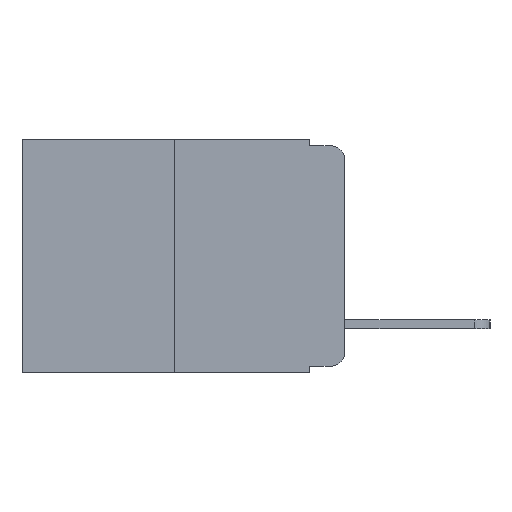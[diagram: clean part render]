
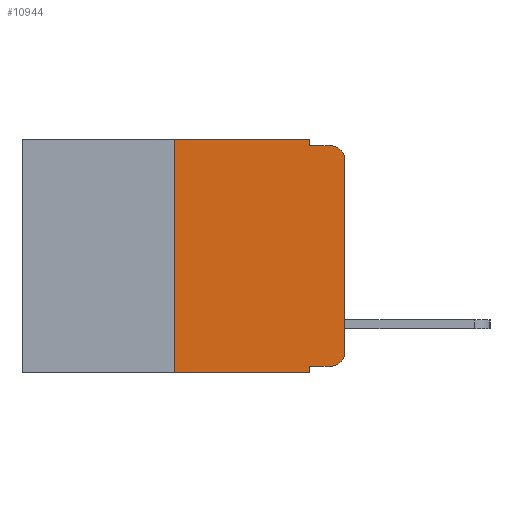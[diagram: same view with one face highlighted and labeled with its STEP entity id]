
A CAD part, left-side view. The second image highlights one B-rep face of the part: STEP entity #10944.
In plain terms, the highlighted planar face has unit normal (-1, 0, 0).
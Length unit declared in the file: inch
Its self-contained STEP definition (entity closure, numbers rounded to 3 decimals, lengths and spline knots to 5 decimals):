
#168 = ORIENTED_EDGE ( 'NONE', *, *, #9440, .F. ) ;
#286 = VERTEX_POINT ( 'NONE', #8980 ) ;
#292 = ORIENTED_EDGE ( 'NONE', *, *, #3671, .F. ) ;
#321 = LINE ( 'NONE', #7393, #3184 ) ;
#363 = VERTEX_POINT ( 'NONE', #466 ) ;
#466 = CARTESIAN_POINT ( 'NONE',  ( 0., 0.051, 0. ) ) ;
#645 = VERTEX_POINT ( 'NONE', #10876 ) ;
#827 = LINE ( 'NONE', #9065, #7703 ) ;
#958 = ORIENTED_EDGE ( 'NONE', *, *, #8987, .T. ) ;
#1052 = ORIENTED_EDGE ( 'NONE', *, *, #4785, .F. ) ;
#1501 = ORIENTED_EDGE ( 'NONE', *, *, #6517, .T. ) ;
#1769 = AXIS2_PLACEMENT_3D ( 'NONE', #6412, #6434, #8892 ) ;
#1824 = ORIENTED_EDGE ( 'NONE', *, *, #7734, .F. ) ;
#2064 = DIRECTION ( 'NONE',  ( 0., 0., -1. ) ) ;
#2206 = LINE ( 'NONE', #8111, #6698 ) ;
#2406 = EDGE_CURVE ( 'NONE', #8271, #8794, #7640, .T. ) ;
#2451 = PLANE ( 'NONE',  #5122 ) ;
#2508 = AXIS2_PLACEMENT_3D ( 'NONE', #6768, #6117, #10990 ) ;
#2649 = ORIENTED_EDGE ( 'NONE', *, *, #7125, .T. ) ;
#2924 = DIRECTION ( 'NONE',  ( 0., -1., 0. ) ) ;
#3184 = VECTOR ( 'NONE', #7811, 39.37008 ) ;
#3581 = CARTESIAN_POINT ( 'NONE',  ( 0., 0.051, -0.343 ) ) ;
#3601 = VECTOR ( 'NONE', #7211, 39.37008 ) ;
#3671 = EDGE_CURVE ( 'NONE', #9602, #286, #4407, .T. ) ;
#3772 = ORIENTED_EDGE ( 'NONE', *, *, #2406, .T. ) ;
#3958 = CIRCLE ( 'NONE', #2508, 0.02 ) ;
#4056 = CIRCLE ( 'NONE', #1769, 0.02 ) ;
#4112 = VECTOR ( 'NONE', #6065, 39.37008 ) ;
#4359 = DIRECTION ( 'NONE',  ( 0., 0., -1. ) ) ;
#4403 = CARTESIAN_POINT ( 'NONE',  ( 0., 0.051, 0. ) ) ;
#4407 = LINE ( 'NONE', #5744, #4112 ) ;
#4785 = EDGE_CURVE ( 'NONE', #8271, #5115, #827, .T. ) ;
#4931 = FACE_OUTER_BOUND ( 'NONE', #7678, .T. ) ;
#5115 = VERTEX_POINT ( 'NONE', #3581 ) ;
#5122 = AXIS2_PLACEMENT_3D ( 'NONE', #8563, #9435, #4359 ) ;
#5390 = VECTOR ( 'NONE', #10019, 39.37008 ) ;
#5720 = VERTEX_POINT ( 'NONE', #8376 ) ;
#5744 = CARTESIAN_POINT ( 'NONE',  ( 0., 0.25, 0. ) ) ;
#5969 = LINE ( 'NONE', #6551, #3601 ) ;
#6052 = DIRECTION ( 'NONE',  ( 0., 0., -1. ) ) ;
#6065 = DIRECTION ( 'NONE',  ( 0., 0., 1. ) ) ;
#6117 = DIRECTION ( 'NONE',  ( -1., 0., 0. ) ) ;
#6412 = CARTESIAN_POINT ( 'NONE',  ( 0., 0.02, -0.03 ) ) ;
#6434 = DIRECTION ( 'NONE',  ( -1., 0., 0. ) ) ;
#6458 = LINE ( 'NONE', #9501, #10564 ) ;
#6517 = EDGE_CURVE ( 'NONE', #8876, #5720, #4056, .T. ) ;
#6551 = CARTESIAN_POINT ( 'NONE',  ( 0., 0.051, -0.01 ) ) ;
#6650 = ORIENTED_EDGE ( 'NONE', *, *, #10384, .T. ) ;
#6672 = ORIENTED_EDGE ( 'NONE', *, *, #10073, .F. ) ;
#6694 = VECTOR ( 'NONE', #2064, 39.37008 ) ;
#6698 = VECTOR ( 'NONE', #2924, 39.37008 ) ;
#6768 = CARTESIAN_POINT ( 'NONE',  ( 0., 0.02, -0.313 ) ) ;
#6860 = CARTESIAN_POINT ( 'NONE',  ( 0., 0.051, -0.01 ) ) ;
#7125 = EDGE_CURVE ( 'NONE', #645, #8876, #321, .T. ) ;
#7211 = DIRECTION ( 'NONE',  ( 0., -1., 0. ) ) ;
#7364 = CARTESIAN_POINT ( 'NONE',  ( 0., 0.051, -0.333 ) ) ;
#7393 = CARTESIAN_POINT ( 'NONE',  ( 0., 0., 0. ) ) ;
#7640 = LINE ( 'NONE', #9647, #5390 ) ;
#7678 = EDGE_LOOP ( 'NONE', ( #2649, #1501, #1824, #168, #6672, #292, #958, #1052, #3772, #6650 ) ) ;
#7703 = VECTOR ( 'NONE', #6052, 39.37008 ) ;
#7734 = EDGE_CURVE ( 'NONE', #10888, #5720, #5969, .T. ) ;
#7810 = DIRECTION ( 'NONE',  ( 0., -1., 0. ) ) ;
#7811 = DIRECTION ( 'NONE',  ( 0., 0., 1. ) ) ;
#8111 = CARTESIAN_POINT ( 'NONE',  ( 0., 0.473, 0. ) ) ;
#8227 = CARTESIAN_POINT ( 'NONE',  ( 0., 0.25, -0.343 ) ) ;
#8263 = CARTESIAN_POINT ( 'NONE',  ( 0., 0.02, -0.333 ) ) ;
#8271 = VERTEX_POINT ( 'NONE', #7364 ) ;
#8376 = CARTESIAN_POINT ( 'NONE',  ( 0., 0.02, -0.01 ) ) ;
#8563 = CARTESIAN_POINT ( 'NONE',  ( 0., 0.473, 0. ) ) ;
#8794 = VERTEX_POINT ( 'NONE', #8263 ) ;
#8876 = VERTEX_POINT ( 'NONE', #11148 ) ;
#8878 = LINE ( 'NONE', #4403, #6694 ) ;
#8892 = DIRECTION ( 'NONE',  ( 0., 0., -1. ) ) ;
#8980 = CARTESIAN_POINT ( 'NONE',  ( 0., 0.25, 0. ) ) ;
#8987 = EDGE_CURVE ( 'NONE', #9602, #5115, #6458, .T. ) ;
#9065 = CARTESIAN_POINT ( 'NONE',  ( 0., 0.051, 0. ) ) ;
#9435 = DIRECTION ( 'NONE',  ( 1., 0., 0. ) ) ;
#9440 = EDGE_CURVE ( 'NONE', #363, #10888, #8878, .T. ) ;
#9501 = CARTESIAN_POINT ( 'NONE',  ( 0., 0.473, -0.343 ) ) ;
#9602 = VERTEX_POINT ( 'NONE', #8227 ) ;
#9647 = CARTESIAN_POINT ( 'NONE',  ( 0., 0.051, -0.333 ) ) ;
#10019 = DIRECTION ( 'NONE',  ( 0., -1., 0. ) ) ;
#10073 = EDGE_CURVE ( 'NONE', #286, #363, #2206, .T. ) ;
#10384 = EDGE_CURVE ( 'NONE', #8794, #645, #3958, .T. ) ;
#10564 = VECTOR ( 'NONE', #7810, 39.37008 ) ;
#10876 = CARTESIAN_POINT ( 'NONE',  ( 0., 0., -0.313 ) ) ;
#10888 = VERTEX_POINT ( 'NONE', #6860 ) ;
#10944 = ADVANCED_FACE ( 'NONE', ( #4931 ), #2451, .F. ) ;
#10990 = DIRECTION ( 'NONE',  ( 0., 0., -1. ) ) ;
#11148 = CARTESIAN_POINT ( 'NONE',  ( 0., 0., -0.03 ) ) ;
